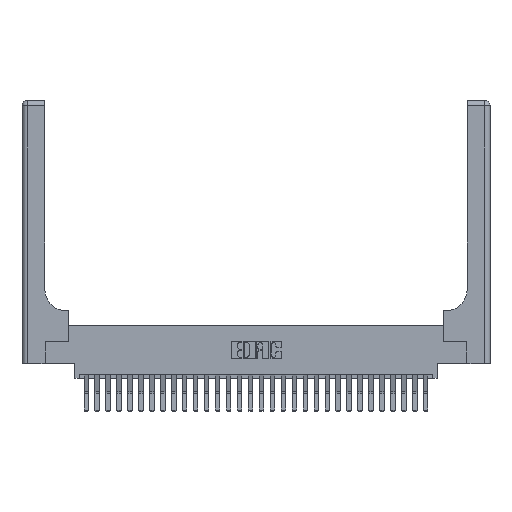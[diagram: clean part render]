
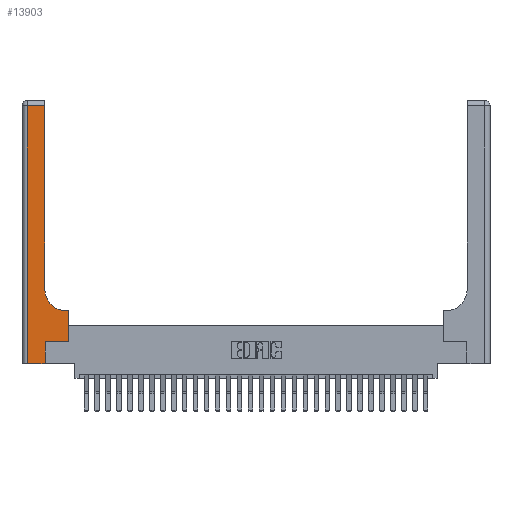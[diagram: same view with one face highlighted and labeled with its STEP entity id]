
A CAD part, top view. The second image highlights one B-rep face of the part: STEP entity #13903.
In plain terms, the highlighted planar face has unit normal (0, 0, 1).
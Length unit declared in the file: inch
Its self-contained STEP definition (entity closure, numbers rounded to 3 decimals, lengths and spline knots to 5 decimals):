
#884 = CARTESIAN_POINT ( 'NONE',  ( 0.51, 0.85, 0.37 ) ) ;
#1151 = VECTOR ( 'NONE', #22090, 39.37008 ) ;
#1377 = LINE ( 'NONE', #16418, #27148 ) ;
#1690 = VERTEX_POINT ( 'NONE', #24508 ) ;
#3867 = CARTESIAN_POINT ( 'NONE',  ( 0., 3., 0.37 ) ) ;
#3889 = ORIENTED_EDGE ( 'NONE', *, *, #7900, .T. ) ;
#4090 = LINE ( 'NONE', #12729, #10363 ) ;
#4149 = LINE ( 'NONE', #27757, #15211 ) ;
#4230 = EDGE_LOOP ( 'NONE', ( #22410, #18934, #3889, #16027, #27444, #17086, #26059, #5126, #8104 ) ) ;
#4338 = EDGE_CURVE ( 'NONE', #5291, #22517, #13325, .T. ) ;
#4559 = DIRECTION ( 'NONE',  ( 0., 1., 0. ) ) ;
#5074 = LINE ( 'NONE', #22398, #8130 ) ;
#5109 = VECTOR ( 'NONE', #11283, 39.37008 ) ;
#5126 = ORIENTED_EDGE ( 'NONE', *, *, #20880, .T. ) ;
#5291 = VERTEX_POINT ( 'NONE', #17522 ) ;
#5968 = AXIS2_PLACEMENT_3D ( 'NONE', #884, #7831, #13962 ) ;
#5990 = PLANE ( 'NONE',  #22909 ) ;
#6410 = FACE_OUTER_BOUND ( 'NONE', #4230, .T. ) ;
#7831 = DIRECTION ( 'NONE',  ( 0., 0., -1. ) ) ;
#7900 = EDGE_CURVE ( 'NONE', #22478, #5291, #15571, .T. ) ;
#8104 = ORIENTED_EDGE ( 'NONE', *, *, #25701, .T. ) ;
#8130 = VECTOR ( 'NONE', #4559, 39.37008 ) ;
#8559 = VERTEX_POINT ( 'NONE', #26152 ) ;
#8655 = CARTESIAN_POINT ( 'NONE',  ( 0., 0., 0.37 ) ) ;
#8836 = CARTESIAN_POINT ( 'NONE',  ( 0.528, 0.25, 0.37 ) ) ;
#9045 = CARTESIAN_POINT ( 'NONE',  ( 0.06, 3., 0.37 ) ) ;
#10185 = VERTEX_POINT ( 'NONE', #8836 ) ;
#10311 = VECTOR ( 'NONE', #15749, 39.37008 ) ;
#10363 = VECTOR ( 'NONE', #19270, 39.37008 ) ;
#10421 = EDGE_CURVE ( 'NONE', #1690, #23945, #19353, .T. ) ;
#10538 = EDGE_CURVE ( 'NONE', #24569, #10185, #11418, .T. ) ;
#10628 = CARTESIAN_POINT ( 'NONE',  ( 0.528, 0.6, 0.37 ) ) ;
#11283 = DIRECTION ( 'NONE',  ( 0., 1., 0. ) ) ;
#11418 = LINE ( 'NONE', #16365, #14667 ) ;
#12729 = CARTESIAN_POINT ( 'NONE',  ( 0.26, 0.6, 0.37 ) ) ;
#13325 = LINE ( 'NONE', #8655, #10311 ) ;
#13842 = EDGE_CURVE ( 'NONE', #23945, #22478, #4149, .T. ) ;
#13903 = ADVANCED_FACE ( 'NONE', ( #6410 ), #5990, .F. ) ;
#13962 = DIRECTION ( 'NONE',  ( 1., 0., 0. ) ) ;
#14667 = VECTOR ( 'NONE', #22750, 39.37008 ) ;
#15211 = VECTOR ( 'NONE', #21619, 39.37008 ) ;
#15527 = CARTESIAN_POINT ( 'NONE',  ( 0.26, 3., 0.37 ) ) ;
#15571 = LINE ( 'NONE', #9045, #1151 ) ;
#15749 = DIRECTION ( 'NONE',  ( 1., 0., 0. ) ) ;
#16027 = ORIENTED_EDGE ( 'NONE', *, *, #4338, .T. ) ;
#16365 = CARTESIAN_POINT ( 'NONE',  ( 0.265, 0.25, 0.37 ) ) ;
#16418 = CARTESIAN_POINT ( 'NONE',  ( 0.265, 0., 0.37 ) ) ;
#16503 = VERTEX_POINT ( 'NONE', #10628 ) ;
#17086 = ORIENTED_EDGE ( 'NONE', *, *, #10538, .T. ) ;
#17522 = CARTESIAN_POINT ( 'NONE',  ( 0.06, 0., 0.37 ) ) ;
#18934 = ORIENTED_EDGE ( 'NONE', *, *, #13842, .T. ) ;
#18948 = CARTESIAN_POINT ( 'NONE',  ( 0.06, 2.94, 0.37 ) ) ;
#19182 = DIRECTION ( 'NONE',  ( 0., 0., -1. ) ) ;
#19270 = DIRECTION ( 'NONE',  ( -1., 0., 0. ) ) ;
#19353 = LINE ( 'NONE', #15527, #5109 ) ;
#20880 = EDGE_CURVE ( 'NONE', #16503, #8559, #4090, .T. ) ;
#20998 = EDGE_CURVE ( 'NONE', #22517, #24569, #1377, .T. ) ;
#21003 = CARTESIAN_POINT ( 'NONE',  ( 0.265, 0., 0.37 ) ) ;
#21026 = CARTESIAN_POINT ( 'NONE',  ( 0.265, 0.25, 0.37 ) ) ;
#21619 = DIRECTION ( 'NONE',  ( -1., 0., 0. ) ) ;
#22090 = DIRECTION ( 'NONE',  ( 0., -1., 0. ) ) ;
#22245 = EDGE_CURVE ( 'NONE', #10185, #16503, #5074, .T. ) ;
#22305 = CIRCLE ( 'NONE', #5968, 0.25 ) ;
#22398 = CARTESIAN_POINT ( 'NONE',  ( 0.528, 0.25, 0.37 ) ) ;
#22410 = ORIENTED_EDGE ( 'NONE', *, *, #10421, .T. ) ;
#22478 = VERTEX_POINT ( 'NONE', #18948 ) ;
#22517 = VERTEX_POINT ( 'NONE', #21003 ) ;
#22750 = DIRECTION ( 'NONE',  ( 1., 0., 0. ) ) ;
#22909 = AXIS2_PLACEMENT_3D ( 'NONE', #3867, #19182, #27901 ) ;
#23945 = VERTEX_POINT ( 'NONE', #24071 ) ;
#24071 = CARTESIAN_POINT ( 'NONE',  ( 0.26, 2.94, 0.37 ) ) ;
#24508 = CARTESIAN_POINT ( 'NONE',  ( 0.26, 0.85, 0.37 ) ) ;
#24569 = VERTEX_POINT ( 'NONE', #21026 ) ;
#25109 = DIRECTION ( 'NONE',  ( 0., 1., 0. ) ) ;
#25701 = EDGE_CURVE ( 'NONE', #8559, #1690, #22305, .T. ) ;
#26059 = ORIENTED_EDGE ( 'NONE', *, *, #22245, .T. ) ;
#26152 = CARTESIAN_POINT ( 'NONE',  ( 0.51, 0.6, 0.37 ) ) ;
#27148 = VECTOR ( 'NONE', #25109, 39.37008 ) ;
#27444 = ORIENTED_EDGE ( 'NONE', *, *, #20998, .T. ) ;
#27757 = CARTESIAN_POINT ( 'NONE',  ( 0., 2.94, 0.37 ) ) ;
#27901 = DIRECTION ( 'NONE',  ( -1., 0., 0. ) ) ;
